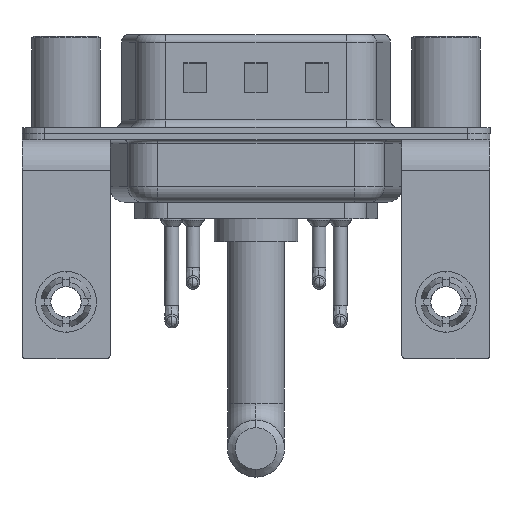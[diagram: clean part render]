
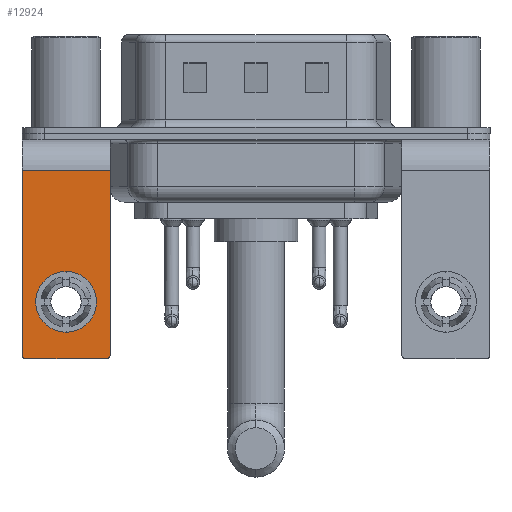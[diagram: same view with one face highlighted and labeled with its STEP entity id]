
A CAD part, front view. The second image highlights one B-rep face of the part: STEP entity #12924.
In plain terms, the highlighted planar face has unit normal (0, -1, 0).
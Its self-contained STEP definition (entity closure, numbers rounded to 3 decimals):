
#630 = CIRCLE ( 'NONE', #7473, 0.25 ) ;
#674 = FACE_BOUND ( 'NONE', #20881, .T. ) ;
#747 = DIRECTION ( 'NONE',  ( 0., 0., 1. ) ) ;
#983 = CARTESIAN_POINT ( 'NONE',  ( 0., -6.25, -11.07 ) ) ;
#1076 = DIRECTION ( 'NONE',  ( 0., 0., 1. ) ) ;
#1132 = VECTOR ( 'NONE', #15953, 1000. ) ;
#1738 = CARTESIAN_POINT ( 'NONE',  ( 2.9, -6.25, -14.8 ) ) ;
#1947 = CARTESIAN_POINT ( 'NONE',  ( 0., -6.25, -9.07 ) ) ;
#2650 = AXIS2_PLACEMENT_3D ( 'NONE', #11178, #7513, #11421 ) ;
#2860 = VERTEX_POINT ( 'NONE', #14122 ) ;
#2922 = DIRECTION ( 'NONE',  ( 0., 1., 0. ) ) ;
#3310 = CARTESIAN_POINT ( 'NONE',  ( 2.9, -6.25, -2.4 ) ) ;
#3353 = VERTEX_POINT ( 'NONE', #6206 ) ;
#3514 = LINE ( 'NONE', #1738, #8393 ) ;
#3613 = LINE ( 'NONE', #12177, #9035 ) ;
#3792 = EDGE_LOOP ( 'NONE', ( #20833, #18689, #14484, #10526, #12621, #8439 ) ) ;
#3945 = AXIS2_PLACEMENT_3D ( 'NONE', #11593, #2922, #18848 ) ;
#4040 = EDGE_CURVE ( 'NONE', #6087, #21633, #4689, .T. ) ;
#4167 = VERTEX_POINT ( 'NONE', #10795 ) ;
#4351 = PLANE ( 'NONE',  #3945 ) ;
#4475 = AXIS2_PLACEMENT_3D ( 'NONE', #983, #18915, #747 ) ;
#4484 = ORIENTED_EDGE ( 'NONE', *, *, #18875, .T. ) ;
#4689 = CIRCLE ( 'NONE', #13785, 2. ) ;
#4712 = FACE_OUTER_BOUND ( 'NONE', #3792, .T. ) ;
#4877 = CARTESIAN_POINT ( 'NONE',  ( -2.9, -6.25, -14.55 ) ) ;
#5312 = VERTEX_POINT ( 'NONE', #4877 ) ;
#5840 = CARTESIAN_POINT ( 'NONE',  ( 2.65, -6.25, -14.55 ) ) ;
#5959 = DIRECTION ( 'NONE',  ( 0., -1., 0. ) ) ;
#6084 = DIRECTION ( 'NONE',  ( 0., 0., 1. ) ) ;
#6087 = VERTEX_POINT ( 'NONE', #1947 ) ;
#6206 = CARTESIAN_POINT ( 'NONE',  ( 2.9, -6.25, -2.4 ) ) ;
#6657 = EDGE_CURVE ( 'NONE', #20111, #4167, #630, .T. ) ;
#6693 = CARTESIAN_POINT ( 'NONE',  ( 2.9, -6.25, -2.4 ) ) ;
#6897 = ORIENTED_EDGE ( 'NONE', *, *, #4040, .T. ) ;
#7211 = CIRCLE ( 'NONE', #2650, 0.25 ) ;
#7473 = AXIS2_PLACEMENT_3D ( 'NONE', #5840, #5959, #6084 ) ;
#7513 = DIRECTION ( 'NONE',  ( 0., -1., 0. ) ) ;
#8247 = VECTOR ( 'NONE', #10559, 1000. ) ;
#8393 = VECTOR ( 'NONE', #16111, 1000. ) ;
#8439 = ORIENTED_EDGE ( 'NONE', *, *, #20421, .T. ) ;
#8442 = DIRECTION ( 'NONE',  ( 0., 1., 0. ) ) ;
#8495 = DIRECTION ( 'NONE',  ( 0., 0., -1. ) ) ;
#9035 = VECTOR ( 'NONE', #8495, 1000. ) ;
#10526 = ORIENTED_EDGE ( 'NONE', *, *, #6657, .T. ) ;
#10559 = DIRECTION ( 'NONE',  ( 0., 0., -1. ) ) ;
#10795 = CARTESIAN_POINT ( 'NONE',  ( 2.9, -6.25, -14.55 ) ) ;
#11178 = CARTESIAN_POINT ( 'NONE',  ( -2.65, -6.25, -14.55 ) ) ;
#11421 = DIRECTION ( 'NONE',  ( 0., 0., 1. ) ) ;
#11593 = CARTESIAN_POINT ( 'NONE',  ( 2.9, -6.25, -2.4 ) ) ;
#12177 = CARTESIAN_POINT ( 'NONE',  ( -2.9, -6.25, -2.4 ) ) ;
#12621 = ORIENTED_EDGE ( 'NONE', *, *, #22576, .F. ) ;
#12924 = ADVANCED_FACE ( 'NONE', ( #674, #4712 ), #4351, .F. ) ;
#13785 = AXIS2_PLACEMENT_3D ( 'NONE', #22813, #8442, #1076 ) ;
#14122 = CARTESIAN_POINT ( 'NONE',  ( -2.65, -6.25, -14.8 ) ) ;
#14484 = ORIENTED_EDGE ( 'NONE', *, *, #21776, .F. ) ;
#15002 = CARTESIAN_POINT ( 'NONE',  ( 2.65, -6.25, -14.8 ) ) ;
#15953 = DIRECTION ( 'NONE',  ( -1., 0., 0. ) ) ;
#16111 = DIRECTION ( 'NONE',  ( -1., 0., 0. ) ) ;
#18488 = EDGE_CURVE ( 'NONE', #21902, #5312, #3613, .T. ) ;
#18689 = ORIENTED_EDGE ( 'NONE', *, *, #20502, .T. ) ;
#18708 = CARTESIAN_POINT ( 'NONE',  ( -2.9, -6.25, -2.4 ) ) ;
#18848 = DIRECTION ( 'NONE',  ( 0., 0., 1. ) ) ;
#18875 = EDGE_CURVE ( 'NONE', #21633, #6087, #20784, .T. ) ;
#18915 = DIRECTION ( 'NONE',  ( 0., 1., 0. ) ) ;
#19584 = LINE ( 'NONE', #3310, #8247 ) ;
#20111 = VERTEX_POINT ( 'NONE', #15002 ) ;
#20421 = EDGE_CURVE ( 'NONE', #3353, #21902, #23431, .T. ) ;
#20502 = EDGE_CURVE ( 'NONE', #5312, #2860, #7211, .T. ) ;
#20784 = CIRCLE ( 'NONE', #4475, 2. ) ;
#20833 = ORIENTED_EDGE ( 'NONE', *, *, #18488, .T. ) ;
#20866 = CARTESIAN_POINT ( 'NONE',  ( 0., -6.25, -13.07 ) ) ;
#20881 = EDGE_LOOP ( 'NONE', ( #4484, #6897 ) ) ;
#21633 = VERTEX_POINT ( 'NONE', #20866 ) ;
#21776 = EDGE_CURVE ( 'NONE', #20111, #2860, #3514, .T. ) ;
#21902 = VERTEX_POINT ( 'NONE', #18708 ) ;
#22576 = EDGE_CURVE ( 'NONE', #3353, #4167, #19584, .T. ) ;
#22813 = CARTESIAN_POINT ( 'NONE',  ( 0., -6.25, -11.07 ) ) ;
#23431 = LINE ( 'NONE', #6693, #1132 ) ;
